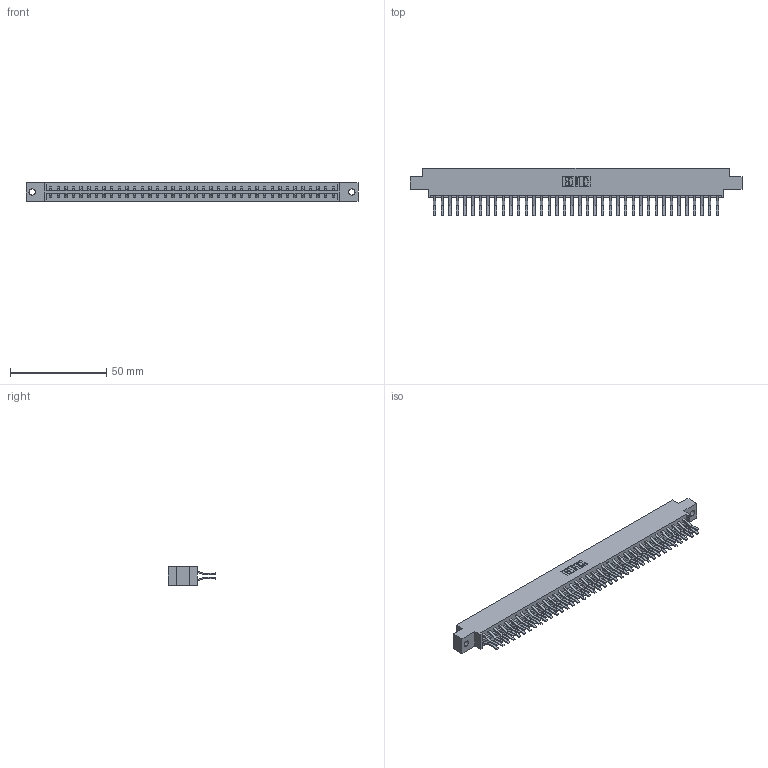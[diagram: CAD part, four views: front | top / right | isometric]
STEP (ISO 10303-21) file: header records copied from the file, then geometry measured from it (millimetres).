
FILE_DESCRIPTION (( 'STEP AP203' ), '1' );
FILE_NAME ('833-076-560-802.STEP', '2020-06-05T19:17:44', ( '' ), ( '' ), 'SwSTEP 2.0', 'SolidWorks 2020', '' );
FILE_SCHEMA (( 'CONFIG_CONTROL_DESIGN' ));
Length unit declared in the file: inch
Products named in the file (3): 345-292-001_560 Tail; 833 Part_Offset - .128 Dia; 833-076-560-802
Assembly tree (77 placements, depth 2):
  833-076-560-802
    833 Part_Offset - .128 Dia
    345-292-001_560 Tail  x76
Bounding box: 172.11 x 24.78 x 9.4 mm (x, y, z)
Volume: 17767.8 mm3; surface area: 22331.5 mm2
Topology: 77 solids, 77 shells, 4222 faces, 12559 edges, 8270 vertices
Faces by surface type: plane 2810, cylinder 1412
Entity records: 25187 total; most frequent: CARTESIAN_POINT 4182, ORIENTED_EDGE 4118, DIRECTION 3583, EDGE_CURVE 2059, LINE 1927, VECTOR 1927, VERTEX_POINT 1370, AXIS2_PLACEMENT_3D 828
